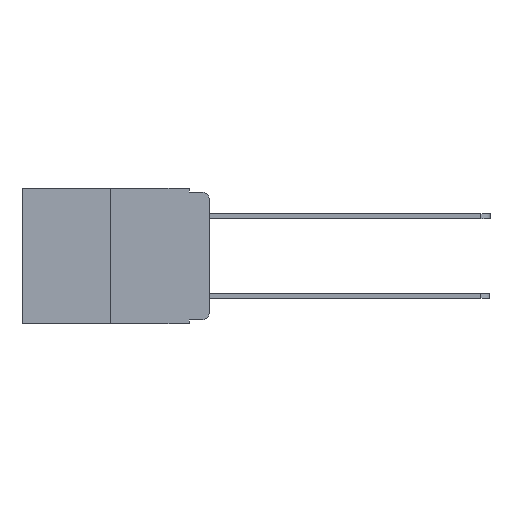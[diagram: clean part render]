
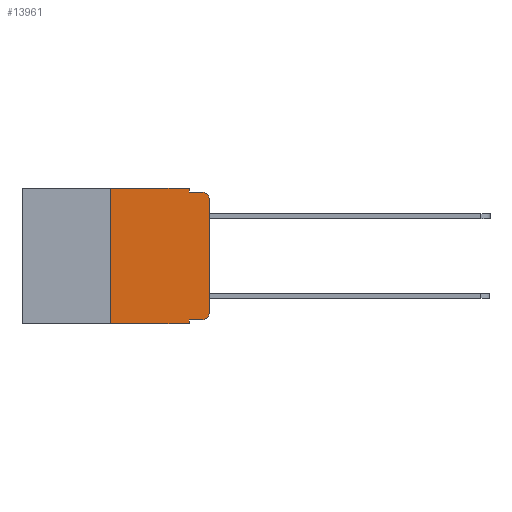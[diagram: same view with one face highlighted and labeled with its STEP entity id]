
A CAD part, left-side view. The second image highlights one B-rep face of the part: STEP entity #13961.
In plain terms, the highlighted planar face has unit normal (-1, 0, 0).
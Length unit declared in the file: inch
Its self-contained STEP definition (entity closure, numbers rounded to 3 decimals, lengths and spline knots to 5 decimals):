
#585 = LINE ( 'NONE', #7312, #14713 ) ;
#676 = ORIENTED_EDGE ( 'NONE', *, *, #3820, .T. ) ;
#1085 = ORIENTED_EDGE ( 'NONE', *, *, #12294, .F. ) ;
#1267 = DIRECTION ( 'NONE',  ( -1., 0., 0. ) ) ;
#1288 = DIRECTION ( 'NONE',  ( 0., 0., -1. ) ) ;
#1309 = DIRECTION ( 'NONE',  ( -1., 0., 0. ) ) ;
#1700 = LINE ( 'NONE', #2990, #4426 ) ;
#1904 = CARTESIAN_POINT ( 'NONE',  ( 0., 0.25, 0. ) ) ;
#1991 = EDGE_CURVE ( 'NONE', #3195, #9761, #15159, .T. ) ;
#2420 = AXIS2_PLACEMENT_3D ( 'NONE', #3395, #1309, #1288 ) ;
#2561 = LINE ( 'NONE', #13241, #12456 ) ;
#2690 = VERTEX_POINT ( 'NONE', #7547 ) ;
#2969 = CARTESIAN_POINT ( 'NONE',  ( 0., 0.051, 0. ) ) ;
#2988 = LINE ( 'NONE', #7970, #3832 ) ;
#2990 = CARTESIAN_POINT ( 'NONE',  ( 0., 0., 0. ) ) ;
#3195 = VERTEX_POINT ( 'NONE', #15675 ) ;
#3221 = CARTESIAN_POINT ( 'NONE',  ( 0., 0.051, 0. ) ) ;
#3395 = CARTESIAN_POINT ( 'NONE',  ( 0., 0.02, -0.03 ) ) ;
#3559 = CIRCLE ( 'NONE', #15715, 0.02 ) ;
#3820 = EDGE_CURVE ( 'NONE', #10301, #2690, #3948, .T. ) ;
#3832 = VECTOR ( 'NONE', #6650, 39.37008 ) ;
#3948 = CIRCLE ( 'NONE', #2420, 0.02 ) ;
#4426 = VECTOR ( 'NONE', #14474, 39.37008 ) ;
#4714 = PLANE ( 'NONE',  #14350 ) ;
#5516 = EDGE_CURVE ( 'NONE', #7133, #2690, #10989, .T. ) ;
#5864 = ORIENTED_EDGE ( 'NONE', *, *, #8801, .T. ) ;
#5992 = CARTESIAN_POINT ( 'NONE',  ( 0., 0.473, 0. ) ) ;
#6225 = DIRECTION ( 'NONE',  ( 0., 0., 1. ) ) ;
#6260 = EDGE_LOOP ( 'NONE', ( #14033, #676, #7692, #11151, #1085, #8098, #11532, #11919, #15549, #5864 ) ) ;
#6434 = DIRECTION ( 'NONE',  ( 0., -1., 0. ) ) ;
#6650 = DIRECTION ( 'NONE',  ( 0., -1., 0. ) ) ;
#6848 = VERTEX_POINT ( 'NONE', #14926 ) ;
#7079 = VERTEX_POINT ( 'NONE', #2969 ) ;
#7133 = VERTEX_POINT ( 'NONE', #8365 ) ;
#7303 = DIRECTION ( 'NONE',  ( 0., 0., -1. ) ) ;
#7312 = CARTESIAN_POINT ( 'NONE',  ( 0., 0.473, -0.343 ) ) ;
#7547 = CARTESIAN_POINT ( 'NONE',  ( 0., 0.02, -0.01 ) ) ;
#7692 = ORIENTED_EDGE ( 'NONE', *, *, #5516, .F. ) ;
#7970 = CARTESIAN_POINT ( 'NONE',  ( 0., 0.473, 0. ) ) ;
#8098 = ORIENTED_EDGE ( 'NONE', *, *, #1991, .F. ) ;
#8149 = VERTEX_POINT ( 'NONE', #11213 ) ;
#8365 = CARTESIAN_POINT ( 'NONE',  ( 0., 0.051, -0.01 ) ) ;
#8596 = EDGE_CURVE ( 'NONE', #3195, #10216, #585, .T. ) ;
#8661 = DIRECTION ( 'NONE',  ( 0., -1., 0. ) ) ;
#8801 = EDGE_CURVE ( 'NONE', #13303, #8149, #3559, .T. ) ;
#9079 = FACE_OUTER_BOUND ( 'NONE', #6260, .T. ) ;
#9169 = CARTESIAN_POINT ( 'NONE',  ( 0., 0.02, -0.313 ) ) ;
#9417 = VECTOR ( 'NONE', #6434, 39.37008 ) ;
#9761 = VERTEX_POINT ( 'NONE', #12163 ) ;
#10216 = VERTEX_POINT ( 'NONE', #10599 ) ;
#10301 = VERTEX_POINT ( 'NONE', #13340 ) ;
#10396 = CARTESIAN_POINT ( 'NONE',  ( 0., 0.051, -0.333 ) ) ;
#10480 = DIRECTION ( 'NONE',  ( 0., 0., -1. ) ) ;
#10599 = CARTESIAN_POINT ( 'NONE',  ( 0., 0.051, -0.343 ) ) ;
#10601 = VECTOR ( 'NONE', #14750, 39.37008 ) ;
#10833 = LINE ( 'NONE', #3221, #13712 ) ;
#10989 = LINE ( 'NONE', #13528, #10601 ) ;
#11151 = ORIENTED_EDGE ( 'NONE', *, *, #15173, .F. ) ;
#11213 = CARTESIAN_POINT ( 'NONE',  ( 0., 0., -0.313 ) ) ;
#11532 = ORIENTED_EDGE ( 'NONE', *, *, #8596, .T. ) ;
#11919 = ORIENTED_EDGE ( 'NONE', *, *, #13033, .F. ) ;
#12163 = CARTESIAN_POINT ( 'NONE',  ( 0., 0.25, 0. ) ) ;
#12294 = EDGE_CURVE ( 'NONE', #9761, #7079, #2988, .T. ) ;
#12409 = EDGE_CURVE ( 'NONE', #8149, #10301, #1700, .T. ) ;
#12456 = VECTOR ( 'NONE', #13294, 39.37008 ) ;
#12640 = CARTESIAN_POINT ( 'NONE',  ( 0., 0.02, -0.333 ) ) ;
#12760 = LINE ( 'NONE', #10396, #9417 ) ;
#13033 = EDGE_CURVE ( 'NONE', #6848, #10216, #2561, .T. ) ;
#13241 = CARTESIAN_POINT ( 'NONE',  ( 0., 0.051, 0. ) ) ;
#13294 = DIRECTION ( 'NONE',  ( 0., 0., -1. ) ) ;
#13303 = VERTEX_POINT ( 'NONE', #12640 ) ;
#13340 = CARTESIAN_POINT ( 'NONE',  ( 0., 0., -0.03 ) ) ;
#13463 = DIRECTION ( 'NONE',  ( 0., 0., -1. ) ) ;
#13528 = CARTESIAN_POINT ( 'NONE',  ( 0., 0.051, -0.01 ) ) ;
#13712 = VECTOR ( 'NONE', #13463, 39.37008 ) ;
#13961 = ADVANCED_FACE ( 'NONE', ( #9079 ), #4714, .F. ) ;
#14033 = ORIENTED_EDGE ( 'NONE', *, *, #12409, .T. ) ;
#14350 = AXIS2_PLACEMENT_3D ( 'NONE', #5992, #14865, #7303 ) ;
#14474 = DIRECTION ( 'NONE',  ( 0., 0., 1. ) ) ;
#14713 = VECTOR ( 'NONE', #8661, 39.37008 ) ;
#14750 = DIRECTION ( 'NONE',  ( 0., -1., 0. ) ) ;
#14778 = VECTOR ( 'NONE', #6225, 39.37008 ) ;
#14865 = DIRECTION ( 'NONE',  ( 1., 0., 0. ) ) ;
#14926 = CARTESIAN_POINT ( 'NONE',  ( 0., 0.051, -0.333 ) ) ;
#15159 = LINE ( 'NONE', #1904, #14778 ) ;
#15173 = EDGE_CURVE ( 'NONE', #7079, #7133, #10833, .T. ) ;
#15549 = ORIENTED_EDGE ( 'NONE', *, *, #16291, .T. ) ;
#15675 = CARTESIAN_POINT ( 'NONE',  ( 0., 0.25, -0.343 ) ) ;
#15715 = AXIS2_PLACEMENT_3D ( 'NONE', #9169, #1267, #10480 ) ;
#16291 = EDGE_CURVE ( 'NONE', #6848, #13303, #12760, .T. ) ;
